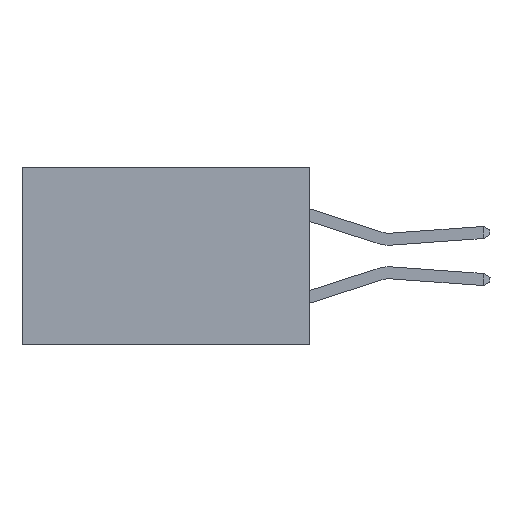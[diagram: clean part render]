
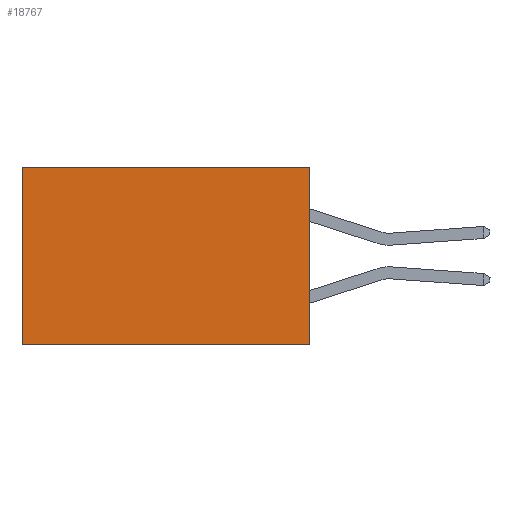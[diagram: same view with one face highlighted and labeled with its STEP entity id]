
A CAD part, left-side view. The second image highlights one B-rep face of the part: STEP entity #18767.
In plain terms, the highlighted planar face has unit normal (-1, 0, 0).
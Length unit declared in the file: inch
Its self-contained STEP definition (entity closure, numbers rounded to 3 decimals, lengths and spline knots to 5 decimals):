
#471 = LINE ( 'NONE', #9330, #12220 ) ;
#781 = LINE ( 'NONE', #6621, #17460 ) ;
#1315 = ORIENTED_EDGE ( 'NONE', *, *, #5212, .T. ) ;
#2117 = FACE_OUTER_BOUND ( 'NONE', #5091, .T. ) ;
#2448 = VERTEX_POINT ( 'NONE', #16537 ) ;
#3887 = VECTOR ( 'NONE', #8577, 39.37008 ) ;
#5091 = EDGE_LOOP ( 'NONE', ( #1315, #15176, #12875, #10737 ) ) ;
#5212 = EDGE_CURVE ( 'NONE', #17273, #2448, #781, .T. ) ;
#5994 = PLANE ( 'NONE',  #9980 ) ;
#6192 = DIRECTION ( 'NONE',  ( 0., 1., 0. ) ) ;
#6356 = CARTESIAN_POINT ( 'NONE',  ( 0.2615, 0., 0. ) ) ;
#6569 = DIRECTION ( 'NONE',  ( 0., 0., -1. ) ) ;
#6621 = CARTESIAN_POINT ( 'NONE',  ( 0.2615, 0.6, -0.37 ) ) ;
#7605 = DIRECTION ( 'NONE',  ( 0., 0., -1. ) ) ;
#7700 = LINE ( 'NONE', #19177, #3887 ) ;
#8577 = DIRECTION ( 'NONE',  ( 0., 0., -1. ) ) ;
#8750 = EDGE_CURVE ( 'NONE', #17296, #17273, #19522, .T. ) ;
#9085 = CARTESIAN_POINT ( 'NONE',  ( 0.2615, 0., -0.37 ) ) ;
#9330 = CARTESIAN_POINT ( 'NONE',  ( 0.2615, 0., -0.37 ) ) ;
#9492 = DIRECTION ( 'NONE',  ( 0., 1., 0. ) ) ;
#9980 = AXIS2_PLACEMENT_3D ( 'NONE', #9085, #16744, #7605 ) ;
#10083 = EDGE_CURVE ( 'NONE', #19499, #2448, #471, .T. ) ;
#10737 = ORIENTED_EDGE ( 'NONE', *, *, #8750, .T. ) ;
#12220 = VECTOR ( 'NONE', #9492, 39.37008 ) ;
#12875 = ORIENTED_EDGE ( 'NONE', *, *, #16217, .F. ) ;
#13079 = CARTESIAN_POINT ( 'NONE',  ( 0.2615, 0., 0. ) ) ;
#15176 = ORIENTED_EDGE ( 'NONE', *, *, #10083, .F. ) ;
#15562 = VECTOR ( 'NONE', #6192, 39.37008 ) ;
#16088 = CARTESIAN_POINT ( 'NONE',  ( 0.2615, 0.6, 0. ) ) ;
#16217 = EDGE_CURVE ( 'NONE', #17296, #19499, #7700, .T. ) ;
#16537 = CARTESIAN_POINT ( 'NONE',  ( 0.2615, 0.6, -0.37 ) ) ;
#16744 = DIRECTION ( 'NONE',  ( 1., 0., 0. ) ) ;
#17273 = VERTEX_POINT ( 'NONE', #16088 ) ;
#17296 = VERTEX_POINT ( 'NONE', #13079 ) ;
#17460 = VECTOR ( 'NONE', #6569, 39.37008 ) ;
#18767 = ADVANCED_FACE ( 'NONE', ( #2117 ), #5994, .F. ) ;
#19177 = CARTESIAN_POINT ( 'NONE',  ( 0.2615, 0., -0.37 ) ) ;
#19499 = VERTEX_POINT ( 'NONE', #19832 ) ;
#19522 = LINE ( 'NONE', #6356, #15562 ) ;
#19832 = CARTESIAN_POINT ( 'NONE',  ( 0.2615, 0., -0.37 ) ) ;
